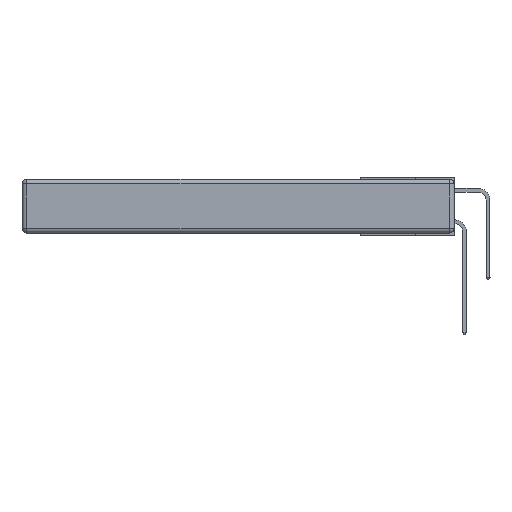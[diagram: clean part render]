
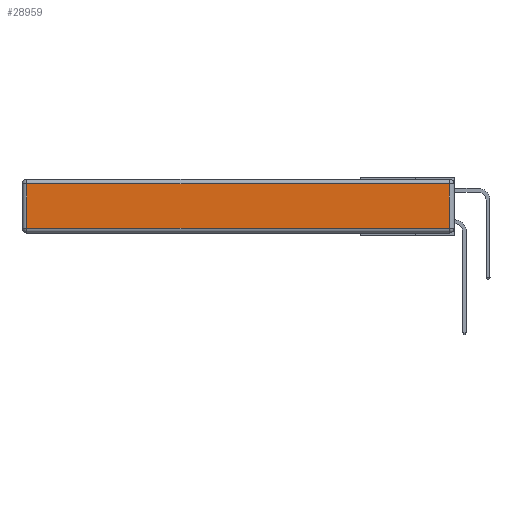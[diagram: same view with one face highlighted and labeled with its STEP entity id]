
A CAD part, left-side view. The second image highlights one B-rep face of the part: STEP entity #28959.
In plain terms, the highlighted planar face has unit normal (-1, 0, 0).
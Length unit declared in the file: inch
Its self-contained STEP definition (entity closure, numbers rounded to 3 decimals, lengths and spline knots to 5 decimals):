
#83 = VERTEX_POINT ( 'NONE', #18003 ) ;
#785 = CARTESIAN_POINT ( 'NONE',  ( 0., 0., -0.313 ) ) ;
#1949 = LINE ( 'NONE', #11704, #29329 ) ;
#2759 = CARTESIAN_POINT ( 'NONE',  ( 0., 2.75, -0.03 ) ) ;
#3277 = LINE ( 'NONE', #21303, #20306 ) ;
#4516 = CARTESIAN_POINT ( 'NONE',  ( 0., 0.03, -0.313 ) ) ;
#5609 = LINE ( 'NONE', #785, #28359 ) ;
#7438 = DIRECTION ( 'NONE',  ( 0., 0., -1. ) ) ;
#7683 = ORIENTED_EDGE ( 'NONE', *, *, #20960, .T. ) ;
#7893 = VERTEX_POINT ( 'NONE', #4516 ) ;
#7978 = CARTESIAN_POINT ( 'NONE',  ( 0., 2.72, -0.03 ) ) ;
#8415 = EDGE_CURVE ( 'NONE', #83, #16521, #27302, .T. ) ;
#9524 = VECTOR ( 'NONE', #11760, 39.37008 ) ;
#11704 = CARTESIAN_POINT ( 'NONE',  ( 0., 2.72, -0.343 ) ) ;
#11760 = DIRECTION ( 'NONE',  ( 0., 1., 0. ) ) ;
#13677 = ORIENTED_EDGE ( 'NONE', *, *, #8415, .T. ) ;
#14498 = DIRECTION ( 'NONE',  ( 0., -1., 0. ) ) ;
#16511 = ORIENTED_EDGE ( 'NONE', *, *, #22776, .T. ) ;
#16521 = VERTEX_POINT ( 'NONE', #7978 ) ;
#18003 = CARTESIAN_POINT ( 'NONE',  ( 0., 0.03, -0.03 ) ) ;
#19176 = EDGE_CURVE ( 'NONE', #16521, #25167, #1949, .T. ) ;
#20306 = VECTOR ( 'NONE', #27971, 39.37008 ) ;
#20960 = EDGE_CURVE ( 'NONE', #7893, #83, #3277, .T. ) ;
#21071 = PLANE ( 'NONE',  #28389 ) ;
#21303 = CARTESIAN_POINT ( 'NONE',  ( 0., 0.03, -0.343 ) ) ;
#22776 = EDGE_CURVE ( 'NONE', #25167, #7893, #5609, .T. ) ;
#22974 = DIRECTION ( 'NONE',  ( 0., 0., 1. ) ) ;
#23376 = DIRECTION ( 'NONE',  ( -1., 0., 0. ) ) ;
#25001 = ORIENTED_EDGE ( 'NONE', *, *, #19176, .T. ) ;
#25167 = VERTEX_POINT ( 'NONE', #28488 ) ;
#27302 = LINE ( 'NONE', #2759, #9524 ) ;
#27730 = CARTESIAN_POINT ( 'NONE',  ( 0., 0., -0.343 ) ) ;
#27971 = DIRECTION ( 'NONE',  ( 0., 0., 1. ) ) ;
#28226 = FACE_OUTER_BOUND ( 'NONE', #29241, .T. ) ;
#28359 = VECTOR ( 'NONE', #14498, 39.37008 ) ;
#28389 = AXIS2_PLACEMENT_3D ( 'NONE', #27730, #23376, #22974 ) ;
#28488 = CARTESIAN_POINT ( 'NONE',  ( 0., 2.72, -0.313 ) ) ;
#28959 = ADVANCED_FACE ( 'NONE', ( #28226 ), #21071, .T. ) ;
#29241 = EDGE_LOOP ( 'NONE', ( #16511, #7683, #13677, #25001 ) ) ;
#29329 = VECTOR ( 'NONE', #7438, 39.37008 ) ;
